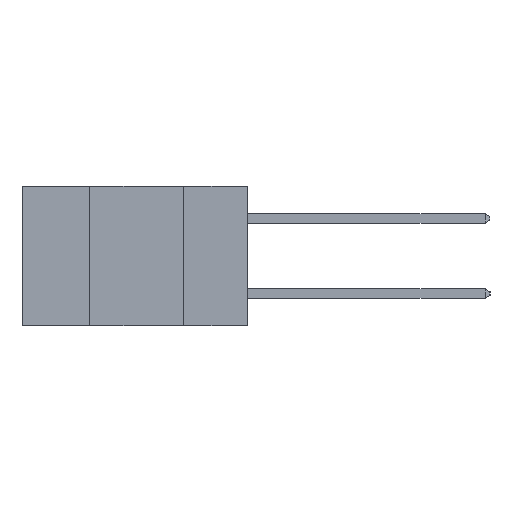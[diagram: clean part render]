
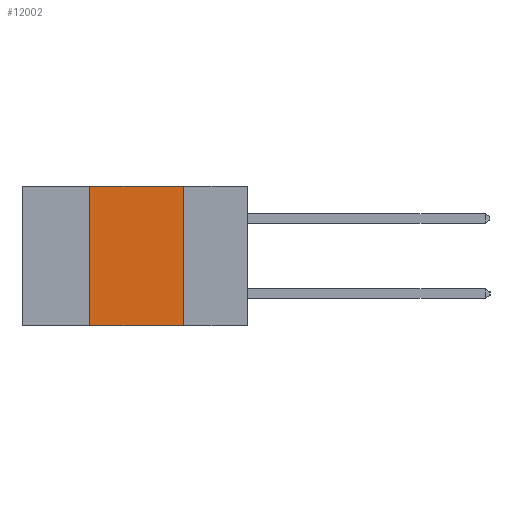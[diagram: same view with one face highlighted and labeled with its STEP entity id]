
A CAD part, left-side view. The second image highlights one B-rep face of the part: STEP entity #12002.
In plain terms, the highlighted planar face has unit normal (-1, 0, 0).
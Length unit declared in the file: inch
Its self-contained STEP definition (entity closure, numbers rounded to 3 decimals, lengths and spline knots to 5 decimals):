
#117 = EDGE_LOOP ( 'NONE', ( #10630, #11026, #3340, #3939 ) ) ;
#216 = FACE_OUTER_BOUND ( 'NONE', #117, .T. ) ;
#583 = AXIS2_PLACEMENT_3D ( 'NONE', #6156, #6153, #6135 ) ;
#659 = CARTESIAN_POINT ( 'NONE',  ( 0., 0.6, 0. ) ) ;
#1403 = DIRECTION ( 'NONE',  ( 0., 0., 1. ) ) ;
#1556 = EDGE_CURVE ( 'NONE', #8905, #11668, #6319, .T. ) ;
#2342 = LINE ( 'NONE', #6620, #5658 ) ;
#3201 = EDGE_CURVE ( 'NONE', #10116, #11668, #2342, .T. ) ;
#3340 = ORIENTED_EDGE ( 'NONE', *, *, #15767, .F. ) ;
#3359 = VECTOR ( 'NONE', #4596, 39.37008 ) ;
#3939 = ORIENTED_EDGE ( 'NONE', *, *, #3201, .T. ) ;
#4596 = DIRECTION ( 'NONE',  ( 0., 0., -1. ) ) ;
#5048 = CARTESIAN_POINT ( 'NONE',  ( 0., 0.17, -0.37 ) ) ;
#5658 = VECTOR ( 'NONE', #7036, 39.37008 ) ;
#5811 = VERTEX_POINT ( 'NONE', #10024 ) ;
#6135 = DIRECTION ( 'NONE',  ( 0., 0., -1. ) ) ;
#6153 = DIRECTION ( 'NONE',  ( 1., 0., 0. ) ) ;
#6156 = CARTESIAN_POINT ( 'NONE',  ( 0., 0.6, 0. ) ) ;
#6253 = PLANE ( 'NONE',  #583 ) ;
#6319 = LINE ( 'NONE', #5048, #3359 ) ;
#6386 = LINE ( 'NONE', #659, #9769 ) ;
#6620 = CARTESIAN_POINT ( 'NONE',  ( 0., 0.6, -0.37 ) ) ;
#7036 = DIRECTION ( 'NONE',  ( 0., -1., 0. ) ) ;
#8243 = DIRECTION ( 'NONE',  ( 0., -1., 0. ) ) ;
#8897 = CARTESIAN_POINT ( 'NONE',  ( 0., 0.17, -0.37 ) ) ;
#8905 = VERTEX_POINT ( 'NONE', #13914 ) ;
#8974 = CARTESIAN_POINT ( 'NONE',  ( 0., 0.42, -0.37 ) ) ;
#9143 = LINE ( 'NONE', #8974, #12793 ) ;
#9769 = VECTOR ( 'NONE', #8243, 39.37008 ) ;
#10024 = CARTESIAN_POINT ( 'NONE',  ( 0., 0.42, 0. ) ) ;
#10116 = VERTEX_POINT ( 'NONE', #12886 ) ;
#10630 = ORIENTED_EDGE ( 'NONE', *, *, #1556, .F. ) ;
#11026 = ORIENTED_EDGE ( 'NONE', *, *, #14730, .F. ) ;
#11668 = VERTEX_POINT ( 'NONE', #8897 ) ;
#12002 = ADVANCED_FACE ( 'NONE', ( #216 ), #6253, .F. ) ;
#12793 = VECTOR ( 'NONE', #1403, 39.37008 ) ;
#12886 = CARTESIAN_POINT ( 'NONE',  ( 0., 0.42, -0.37 ) ) ;
#13914 = CARTESIAN_POINT ( 'NONE',  ( 0., 0.17, 0. ) ) ;
#14730 = EDGE_CURVE ( 'NONE', #5811, #8905, #6386, .T. ) ;
#15767 = EDGE_CURVE ( 'NONE', #10116, #5811, #9143, .T. ) ;
